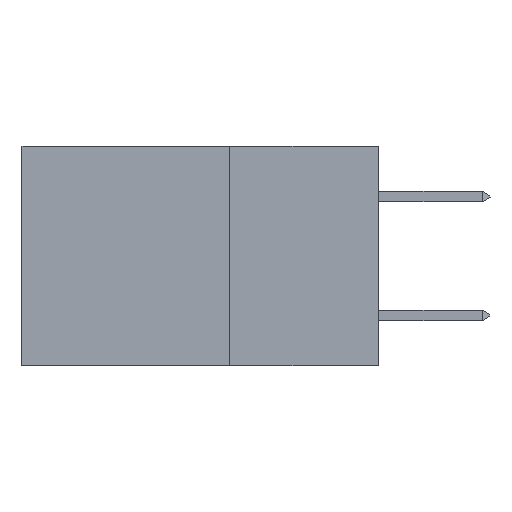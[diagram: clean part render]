
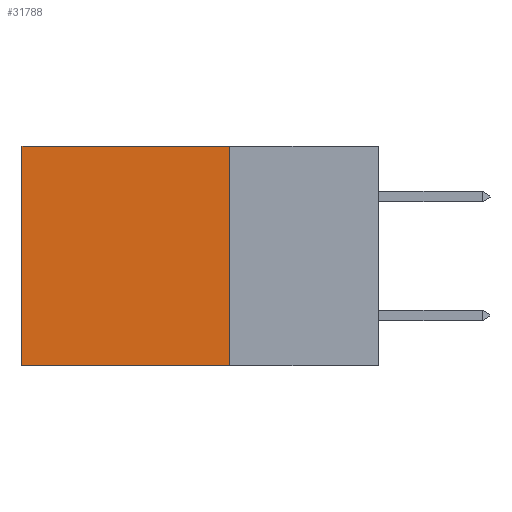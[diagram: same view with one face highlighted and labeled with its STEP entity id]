
A CAD part, left-side view. The second image highlights one B-rep face of the part: STEP entity #31788.
In plain terms, the highlighted planar face has unit normal (-1, 0, 0).
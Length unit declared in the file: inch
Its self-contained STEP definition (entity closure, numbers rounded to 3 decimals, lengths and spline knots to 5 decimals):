
#1145 = EDGE_CURVE ( 'NONE', #31929, #9210, #29604, .T. ) ;
#3493 = DIRECTION ( 'NONE',  ( 0., 1., 0. ) ) ;
#8046 = CARTESIAN_POINT ( 'NONE',  ( 0.298, 0.25, 0. ) ) ;
#8589 = CARTESIAN_POINT ( 'NONE',  ( 0.298, 0.25, -0.37 ) ) ;
#9210 = VERTEX_POINT ( 'NONE', #9517 ) ;
#9517 = CARTESIAN_POINT ( 'NONE',  ( 0.298, 0.6, 0. ) ) ;
#9927 = VECTOR ( 'NONE', #24616, 39.37008 ) ;
#10410 = CARTESIAN_POINT ( 'NONE',  ( 0.298, 0.6, 0. ) ) ;
#11179 = FACE_OUTER_BOUND ( 'NONE', #18279, .T. ) ;
#11652 = ORIENTED_EDGE ( 'NONE', *, *, #1145, .T. ) ;
#12163 = VECTOR ( 'NONE', #28617, 39.37008 ) ;
#13441 = CARTESIAN_POINT ( 'NONE',  ( 0.298, 0.25, 0. ) ) ;
#13974 = VECTOR ( 'NONE', #25835, 39.37008 ) ;
#13975 = CARTESIAN_POINT ( 'NONE',  ( 0.298, 0.25, -0.37 ) ) ;
#14204 = LINE ( 'NONE', #8589, #20227 ) ;
#15467 = EDGE_CURVE ( 'NONE', #9210, #21902, #20812, .T. ) ;
#15995 = DIRECTION ( 'NONE',  ( 0., 0., -1. ) ) ;
#17339 = CARTESIAN_POINT ( 'NONE',  ( 0.298, 0.6, -0.37 ) ) ;
#17666 = EDGE_CURVE ( 'NONE', #31929, #22382, #20655, .T. ) ;
#17859 = EDGE_CURVE ( 'NONE', #22382, #21902, #14204, .T. ) ;
#18279 = EDGE_LOOP ( 'NONE', ( #20375, #20931, #30273, #11652 ) ) ;
#20227 = VECTOR ( 'NONE', #3493, 39.37008 ) ;
#20375 = ORIENTED_EDGE ( 'NONE', *, *, #15467, .T. ) ;
#20655 = LINE ( 'NONE', #8046, #12163 ) ;
#20812 = LINE ( 'NONE', #10410, #13974 ) ;
#20931 = ORIENTED_EDGE ( 'NONE', *, *, #17859, .F. ) ;
#21902 = VERTEX_POINT ( 'NONE', #17339 ) ;
#22382 = VERTEX_POINT ( 'NONE', #13975 ) ;
#23545 = AXIS2_PLACEMENT_3D ( 'NONE', #13441, #31351, #15995 ) ;
#24444 = CARTESIAN_POINT ( 'NONE',  ( 0.298, 0.25, 0. ) ) ;
#24616 = DIRECTION ( 'NONE',  ( 0., 1., 0. ) ) ;
#25835 = DIRECTION ( 'NONE',  ( 0., 0., -1. ) ) ;
#26057 = CARTESIAN_POINT ( 'NONE',  ( 0.298, 0.25, 0. ) ) ;
#28617 = DIRECTION ( 'NONE',  ( 0., 0., -1. ) ) ;
#28808 = PLANE ( 'NONE',  #23545 ) ;
#29604 = LINE ( 'NONE', #26057, #9927 ) ;
#30273 = ORIENTED_EDGE ( 'NONE', *, *, #17666, .F. ) ;
#31351 = DIRECTION ( 'NONE',  ( 1., 0., 0. ) ) ;
#31788 = ADVANCED_FACE ( 'NONE', ( #11179 ), #28808, .F. ) ;
#31929 = VERTEX_POINT ( 'NONE', #24444 ) ;
